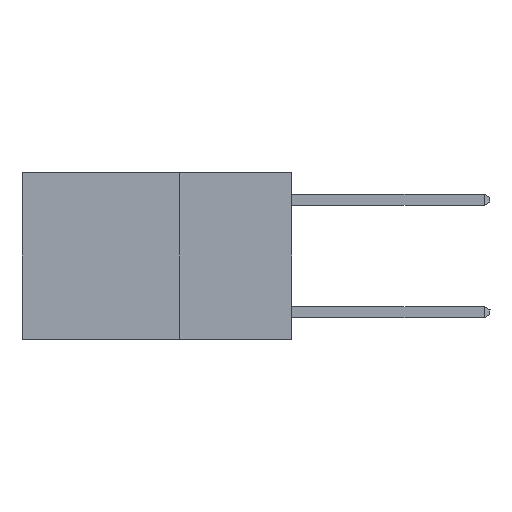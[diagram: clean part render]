
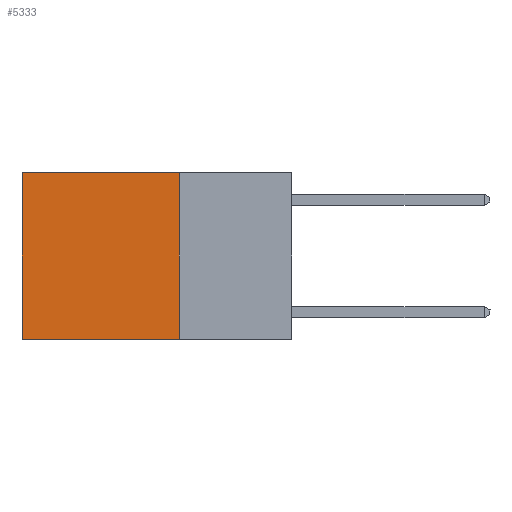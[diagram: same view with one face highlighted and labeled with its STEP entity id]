
A CAD part, left-side view. The second image highlights one B-rep face of the part: STEP entity #5333.
In plain terms, the highlighted planar face has unit normal (-1, 0, 0).
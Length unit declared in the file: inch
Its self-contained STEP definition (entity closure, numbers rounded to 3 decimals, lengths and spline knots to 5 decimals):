
#13 = CARTESIAN_POINT ( 'NONE',  ( 0.2625, 0.25, 0. ) ) ;
#248 = EDGE_CURVE ( 'NONE', #1662, #11351, #9886, .T. ) ;
#401 = ORIENTED_EDGE ( 'NONE', *, *, #7337, .F. ) ;
#487 = DIRECTION ( 'NONE',  ( 0., 0., -1. ) ) ;
#570 = CARTESIAN_POINT ( 'NONE',  ( 0.2625, 0.25, -0.37 ) ) ;
#668 = ORIENTED_EDGE ( 'NONE', *, *, #5631, .T. ) ;
#1162 = AXIS2_PLACEMENT_3D ( 'NONE', #10273, #6115, #487 ) ;
#1495 = VECTOR ( 'NONE', #3126, 39.37008 ) ;
#1662 = VERTEX_POINT ( 'NONE', #10942 ) ;
#2077 = VERTEX_POINT ( 'NONE', #4408 ) ;
#2432 = FACE_OUTER_BOUND ( 'NONE', #10140, .T. ) ;
#2475 = VERTEX_POINT ( 'NONE', #5292 ) ;
#2556 = ORIENTED_EDGE ( 'NONE', *, *, #248, .F. ) ;
#3126 = DIRECTION ( 'NONE',  ( 0., 0., -1. ) ) ;
#3898 = LINE ( 'NONE', #9390, #1495 ) ;
#3957 = LINE ( 'NONE', #7836, #8555 ) ;
#4408 = CARTESIAN_POINT ( 'NONE',  ( 0.2625, 0.6, 0. ) ) ;
#4999 = VECTOR ( 'NONE', #5634, 39.37008 ) ;
#5292 = CARTESIAN_POINT ( 'NONE',  ( 0.2625, 0.6, -0.37 ) ) ;
#5333 = ADVANCED_FACE ( 'NONE', ( #2432 ), #11070, .F. ) ;
#5627 = LINE ( 'NONE', #10902, #7743 ) ;
#5631 = EDGE_CURVE ( 'NONE', #1662, #2077, #3957, .T. ) ;
#5634 = DIRECTION ( 'NONE',  ( 0., 0., -1. ) ) ;
#6115 = DIRECTION ( 'NONE',  ( 1., 0., 0. ) ) ;
#6993 = DIRECTION ( 'NONE',  ( 0., 1., 0. ) ) ;
#7337 = EDGE_CURVE ( 'NONE', #11351, #2475, #5627, .T. ) ;
#7743 = VECTOR ( 'NONE', #9303, 39.37008 ) ;
#7836 = CARTESIAN_POINT ( 'NONE',  ( 0.2625, 0.25, 0. ) ) ;
#8317 = EDGE_CURVE ( 'NONE', #2077, #2475, #3898, .T. ) ;
#8555 = VECTOR ( 'NONE', #6993, 39.37008 ) ;
#9303 = DIRECTION ( 'NONE',  ( 0., 1., 0. ) ) ;
#9390 = CARTESIAN_POINT ( 'NONE',  ( 0.2625, 0.6, 0. ) ) ;
#9886 = LINE ( 'NONE', #13, #4999 ) ;
#10140 = EDGE_LOOP ( 'NONE', ( #10549, #401, #2556, #668 ) ) ;
#10273 = CARTESIAN_POINT ( 'NONE',  ( 0.2625, 0.25, 0. ) ) ;
#10549 = ORIENTED_EDGE ( 'NONE', *, *, #8317, .T. ) ;
#10902 = CARTESIAN_POINT ( 'NONE',  ( 0.2625, 0.25, -0.37 ) ) ;
#10942 = CARTESIAN_POINT ( 'NONE',  ( 0.2625, 0.25, 0. ) ) ;
#11070 = PLANE ( 'NONE',  #1162 ) ;
#11351 = VERTEX_POINT ( 'NONE', #570 ) ;
